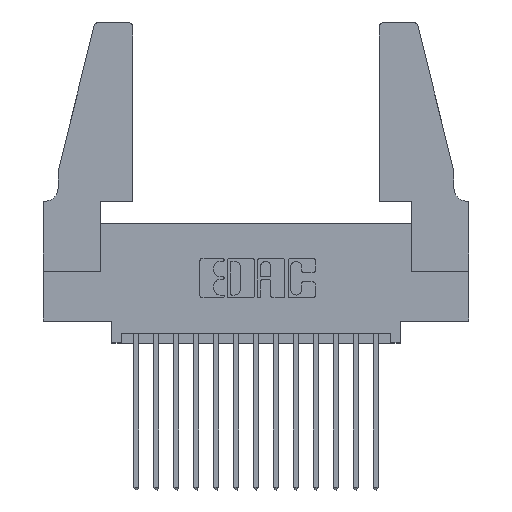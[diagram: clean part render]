
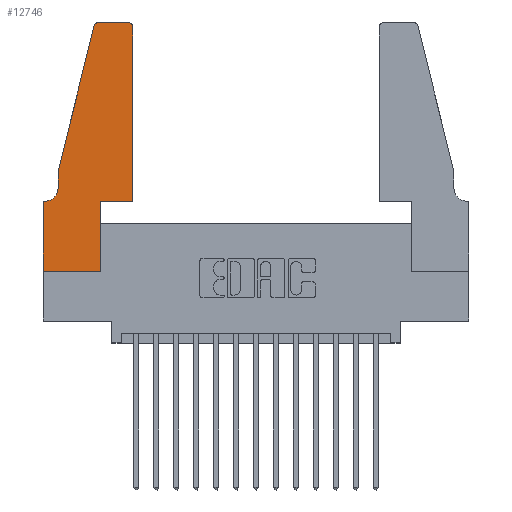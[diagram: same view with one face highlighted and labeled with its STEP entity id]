
A CAD part, top view. The second image highlights one B-rep face of the part: STEP entity #12746.
In plain terms, the highlighted planar face has unit normal (0, 0, 1).
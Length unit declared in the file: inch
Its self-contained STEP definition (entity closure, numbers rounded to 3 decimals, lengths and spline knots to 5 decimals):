
#36 = VECTOR ( 'NONE', #10422, 39.37008 ) ;
#146 = ORIENTED_EDGE ( 'NONE', *, *, #4236, .T. ) ;
#504 = CARTESIAN_POINT ( 'NONE',  ( 0.0755, 0.5, 0.37 ) ) ;
#744 = ORIENTED_EDGE ( 'NONE', *, *, #10711, .T. ) ;
#928 = DIRECTION ( 'NONE',  ( 1., 0., 0. ) ) ;
#970 = DIRECTION ( 'NONE',  ( 0., 0., 1. ) ) ;
#1015 = CARTESIAN_POINT ( 'NONE',  ( 0.284, 1.22, 0.37 ) ) ;
#1088 = CARTESIAN_POINT ( 'NONE',  ( 0.2605, 1.25, 0.37 ) ) ;
#1326 = CARTESIAN_POINT ( 'NONE',  ( 0.2865, 0.35, 0.37 ) ) ;
#1454 = CARTESIAN_POINT ( 'NONE',  ( 0.2865, 0.35, 0.37 ) ) ;
#1572 = EDGE_CURVE ( 'NONE', #2223, #9110, #9978, .T. ) ;
#1696 = VERTEX_POINT ( 'NONE', #3358 ) ;
#1877 = CARTESIAN_POINT ( 'NONE',  ( 0., 0., 0.37 ) ) ;
#2223 = VERTEX_POINT ( 'NONE', #7980 ) ;
#2323 = DIRECTION ( 'NONE',  ( 0., 0., 1. ) ) ;
#2372 = DIRECTION ( 'NONE',  ( 1., 0., 0. ) ) ;
#2535 = CARTESIAN_POINT ( 'NONE',  ( 0.0055, 0.35, 0.37 ) ) ;
#2918 = CARTESIAN_POINT ( 'NONE',  ( 0., 0.35, 0.37 ) ) ;
#2955 = VERTEX_POINT ( 'NONE', #16265 ) ;
#2966 = CIRCLE ( 'NONE', #5388, 0.03 ) ;
#3058 = ORIENTED_EDGE ( 'NONE', *, *, #3568, .T. ) ;
#3358 = CARTESIAN_POINT ( 'NONE',  ( 0.4505, 0.35, 0.37 ) ) ;
#3434 = VECTOR ( 'NONE', #15659, 39.37008 ) ;
#3568 = EDGE_CURVE ( 'NONE', #2955, #13850, #3587, .T. ) ;
#3587 = CIRCLE ( 'NONE', #8807, 0.03 ) ;
#3713 = CARTESIAN_POINT ( 'NONE',  ( 0., 0., 0.37 ) ) ;
#4021 = FACE_OUTER_BOUND ( 'NONE', #9239, .T. ) ;
#4108 = ORIENTED_EDGE ( 'NONE', *, *, #15845, .T. ) ;
#4236 = EDGE_CURVE ( 'NONE', #4390, #2955, #14538, .T. ) ;
#4270 = DIRECTION ( 'NONE',  ( 1., 0., 0. ) ) ;
#4274 = CARTESIAN_POINT ( 'NONE',  ( 0., 0., 0.37 ) ) ;
#4390 = VERTEX_POINT ( 'NONE', #13014 ) ;
#4501 = CARTESIAN_POINT ( 'NONE',  ( 0.0055, 0.42, 0.37 ) ) ;
#4616 = AXIS2_PLACEMENT_3D ( 'NONE', #4501, #13190, #5754 ) ;
#4970 = ORIENTED_EDGE ( 'NONE', *, *, #8822, .T. ) ;
#5091 = VECTOR ( 'NONE', #12120, 39.37008 ) ;
#5202 = CARTESIAN_POINT ( 'NONE',  ( 0.4505, 0.35, 0.37 ) ) ;
#5388 = AXIS2_PLACEMENT_3D ( 'NONE', #10006, #2323, #11239 ) ;
#5486 = LINE ( 'NONE', #5885, #5091 ) ;
#5738 = CARTESIAN_POINT ( 'NONE',  ( 0.0755, 0.35, 0.37 ) ) ;
#5754 = DIRECTION ( 'NONE',  ( -1., 0., 0. ) ) ;
#5885 = CARTESIAN_POINT ( 'NONE',  ( 0.0755, 0.5, 0.37 ) ) ;
#6352 = ORIENTED_EDGE ( 'NONE', *, *, #9610, .T. ) ;
#6461 = DIRECTION ( 'NONE',  ( 0., 1., 0. ) ) ;
#6509 = VECTOR ( 'NONE', #2372, 39.37008 ) ;
#6893 = VERTEX_POINT ( 'NONE', #504 ) ;
#7723 = ORIENTED_EDGE ( 'NONE', *, *, #15720, .T. ) ;
#7980 = CARTESIAN_POINT ( 'NONE',  ( 0.2865, 0., 0.37 ) ) ;
#8381 = VECTOR ( 'NONE', #14228, 39.37008 ) ;
#8542 = CARTESIAN_POINT ( 'NONE',  ( 0.0755, 0.5, 0.37 ) ) ;
#8547 = AXIS2_PLACEMENT_3D ( 'NONE', #2918, #11757, #4270 ) ;
#8807 = AXIS2_PLACEMENT_3D ( 'NONE', #1015, #970, #928 ) ;
#8822 = EDGE_CURVE ( 'NONE', #12159, #13876, #16330, .T. ) ;
#9110 = VERTEX_POINT ( 'NONE', #1326 ) ;
#9239 = EDGE_LOOP ( 'NONE', ( #146, #3058, #744, #7723, #12959, #4970, #11963, #16091, #12340, #6352, #9821, #4108 ) ) ;
#9359 = VERTEX_POINT ( 'NONE', #15646 ) ;
#9610 = EDGE_CURVE ( 'NONE', #9110, #1696, #16387, .T. ) ;
#9821 = ORIENTED_EDGE ( 'NONE', *, *, #11584, .T. ) ;
#9970 = EDGE_CURVE ( 'NONE', #13800, #12159, #13872, .T. ) ;
#9978 = LINE ( 'NONE', #1454, #36 ) ;
#10006 = CARTESIAN_POINT ( 'NONE',  ( 0.4205, 1.22, 0.37 ) ) ;
#10422 = DIRECTION ( 'NONE',  ( 0., 1., 0. ) ) ;
#10543 = PLANE ( 'NONE',  #8547 ) ;
#10711 = EDGE_CURVE ( 'NONE', #13850, #6893, #5486, .T. ) ;
#11239 = DIRECTION ( 'NONE',  ( 1., 0., 0. ) ) ;
#11299 = LINE ( 'NONE', #8542, #14555 ) ;
#11584 = EDGE_CURVE ( 'NONE', #1696, #9359, #12103, .T. ) ;
#11757 = DIRECTION ( 'NONE',  ( 0., 0., 1. ) ) ;
#11963 = ORIENTED_EDGE ( 'NONE', *, *, #16123, .T. ) ;
#12061 = EDGE_CURVE ( 'NONE', #12890, #2223, #14574, .T. ) ;
#12103 = LINE ( 'NONE', #5202, #15352 ) ;
#12120 = DIRECTION ( 'NONE',  ( -0.239, -0.971, 0. ) ) ;
#12159 = VERTEX_POINT ( 'NONE', #2535 ) ;
#12340 = ORIENTED_EDGE ( 'NONE', *, *, #1572, .T. ) ;
#12746 = ADVANCED_FACE ( 'NONE', ( #4021 ), #10543, .T. ) ;
#12750 = CARTESIAN_POINT ( 'NONE',  ( 0.0755, 0.42, 0.37 ) ) ;
#12846 = CARTESIAN_POINT ( 'NONE',  ( 0.25487, 1.22718, 0.37 ) ) ;
#12890 = VERTEX_POINT ( 'NONE', #1877 ) ;
#12959 = ORIENTED_EDGE ( 'NONE', *, *, #9970, .T. ) ;
#13014 = CARTESIAN_POINT ( 'NONE',  ( 0.4205, 1.25, 0.37 ) ) ;
#13190 = DIRECTION ( 'NONE',  ( 0., 0., -1. ) ) ;
#13713 = DIRECTION ( 'NONE',  ( 1., 0., 0. ) ) ;
#13800 = VERTEX_POINT ( 'NONE', #12750 ) ;
#13850 = VERTEX_POINT ( 'NONE', #12846 ) ;
#13872 = CIRCLE ( 'NONE', #4616, 0.07 ) ;
#13876 = VERTEX_POINT ( 'NONE', #14136 ) ;
#14136 = CARTESIAN_POINT ( 'NONE',  ( 0., 0.35, 0.37 ) ) ;
#14150 = VECTOR ( 'NONE', #16241, 39.37008 ) ;
#14186 = VECTOR ( 'NONE', #13713, 39.37008 ) ;
#14228 = DIRECTION ( 'NONE',  ( 0., -1., 0. ) ) ;
#14538 = LINE ( 'NONE', #1088, #14150 ) ;
#14540 = LINE ( 'NONE', #4274, #8381 ) ;
#14555 = VECTOR ( 'NONE', #15906, 39.37008 ) ;
#14574 = LINE ( 'NONE', #3713, #14186 ) ;
#15352 = VECTOR ( 'NONE', #6461, 39.37008 ) ;
#15646 = CARTESIAN_POINT ( 'NONE',  ( 0.4505, 1.22, 0.37 ) ) ;
#15659 = DIRECTION ( 'NONE',  ( -1., 0., 0. ) ) ;
#15720 = EDGE_CURVE ( 'NONE', #6893, #13800, #11299, .T. ) ;
#15845 = EDGE_CURVE ( 'NONE', #9359, #4390, #2966, .T. ) ;
#15906 = DIRECTION ( 'NONE',  ( 0., -1., 0. ) ) ;
#16091 = ORIENTED_EDGE ( 'NONE', *, *, #12061, .T. ) ;
#16123 = EDGE_CURVE ( 'NONE', #13876, #12890, #14540, .T. ) ;
#16156 = CARTESIAN_POINT ( 'NONE',  ( 0.4505, 0.35, 0.37 ) ) ;
#16241 = DIRECTION ( 'NONE',  ( -1., 0., 0. ) ) ;
#16265 = CARTESIAN_POINT ( 'NONE',  ( 0.284, 1.25, 0.37 ) ) ;
#16330 = LINE ( 'NONE', #5738, #3434 ) ;
#16387 = LINE ( 'NONE', #16156, #6509 ) ;
